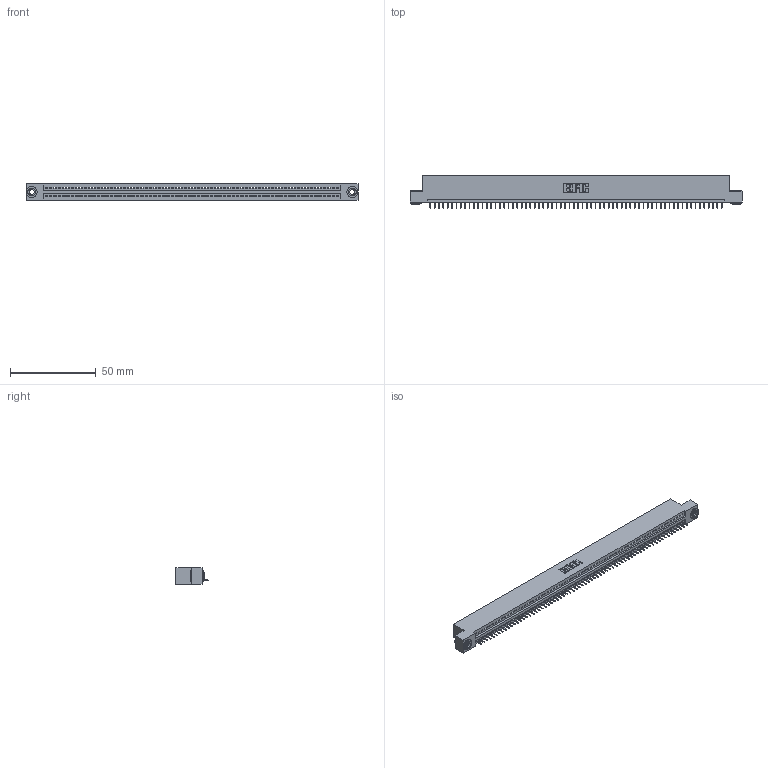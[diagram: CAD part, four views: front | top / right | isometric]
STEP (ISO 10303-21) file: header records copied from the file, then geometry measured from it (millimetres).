
FILE_DESCRIPTION (( 'STEP AP203' ), '1' );
FILE_NAME ('345-068-525-103.STEP', '2020-09-21T05:20:31', ( '' ), ( '' ), 'SwSTEP 2.0', 'SolidWorks 2020', '' );
FILE_SCHEMA (( 'CONFIG_CONTROL_DESIGN' ));
Length unit declared in the file: inch
Products named in the file (4): 345-250-002_345-250-002-102; 345-292-001_345-293-125; 345 Part_Flush Mounting Lugs - 0.156 Dia-TH; 345-068-525-103
Assembly tree (71 placements, depth 2):
  345-068-525-103
    345 Part_Flush Mounting Lugs - 0.156 Dia-TH
    345-292-001_345-293-125  x68
    345-250-002_345-250-002-102  x2
Bounding box: 193.93 x 18.72 x 9.4 mm (x, y, z)
Volume: 18374.3 mm3; surface area: 24059.8 mm2
Topology: 71 solids, 71 shells, 4380 faces, 12657 edges, 8162 vertices
Faces by surface type: plane 3218, cylinder 1154, cone 8
Entity records: 48402 total; most frequent: CARTESIAN_POINT 8359, ORIENTED_EDGE 8354, DIRECTION 7295, EDGE_CURVE 4177, LINE 3753, VECTOR 3753, VERTEX_POINT 2778, AXIS2_PLACEMENT_3D 1771
